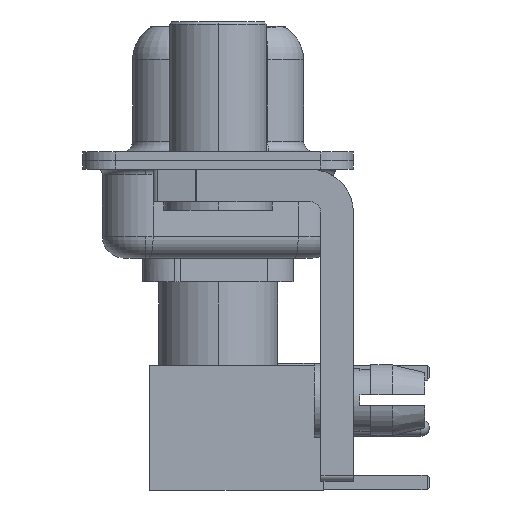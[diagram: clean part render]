
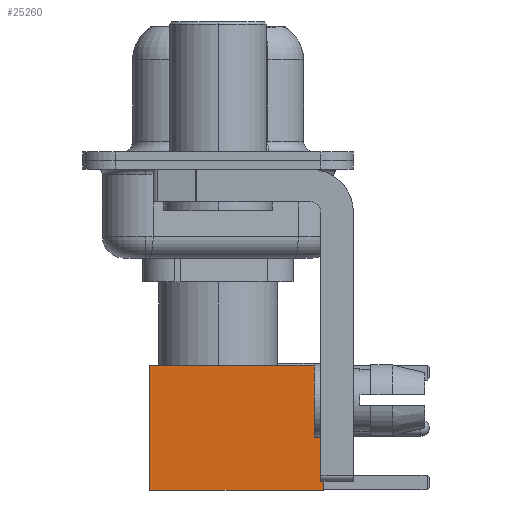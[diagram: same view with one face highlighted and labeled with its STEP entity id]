
A CAD part, left-side view. The second image highlights one B-rep face of the part: STEP entity #25260.
In plain terms, the highlighted face is planar.
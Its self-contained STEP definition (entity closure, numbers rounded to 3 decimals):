
#2645 = ORIENTED_EDGE ( 'NONE', *, *, #20282, .T. ) ;
#3722 = LINE ( 'NONE', #12527, #17031 ) ;
#4280 = CARTESIAN_POINT ( 'NONE',  ( 2.875, 2.875, 0. ) ) ;
#4749 = EDGE_CURVE ( 'NONE', #17745, #22793, #21740, .T. ) ;
#5296 = CARTESIAN_POINT ( 'NONE',  ( -2.875, 2.875, 8. ) ) ;
#5367 = CARTESIAN_POINT ( 'NONE',  ( 2.875, 2.875, 0. ) ) ;
#5919 = FACE_OUTER_BOUND ( 'NONE', #9492, .T. ) ;
#6090 = DIRECTION ( 'NONE',  ( 0., 0., -1. ) ) ;
#7211 = DIRECTION ( 'NONE',  ( -1., 0., 0. ) ) ;
#8745 = DIRECTION ( 'NONE',  ( 0., 0., 1. ) ) ;
#9492 = EDGE_LOOP ( 'NONE', ( #13717, #2645, #17162, #9732 ) ) ;
#9615 = EDGE_CURVE ( 'NONE', #10635, #19269, #24761, .T. ) ;
#9732 = ORIENTED_EDGE ( 'NONE', *, *, #21240, .F. ) ;
#9874 = CARTESIAN_POINT ( 'NONE',  ( 2.875, 2.875, 8. ) ) ;
#10264 = AXIS2_PLACEMENT_3D ( 'NONE', #5367, #14451, #8745 ) ;
#10635 = VERTEX_POINT ( 'NONE', #9874 ) ;
#12228 = VECTOR ( 'NONE', #6090, 1000. ) ;
#12253 = CARTESIAN_POINT ( 'NONE',  ( -2.875, 2.875, 0. ) ) ;
#12527 = CARTESIAN_POINT ( 'NONE',  ( 0., 2.875, 8. ) ) ;
#13603 = CARTESIAN_POINT ( 'NONE',  ( 0., 2.875, 0. ) ) ;
#13717 = ORIENTED_EDGE ( 'NONE', *, *, #9615, .T. ) ;
#14451 = DIRECTION ( 'NONE',  ( 0., 1., 0. ) ) ;
#15535 = CARTESIAN_POINT ( 'NONE',  ( -2.875, 2.875, 0. ) ) ;
#17031 = VECTOR ( 'NONE', #21645, 1000. ) ;
#17162 = ORIENTED_EDGE ( 'NONE', *, *, #4749, .F. ) ;
#17745 = VERTEX_POINT ( 'NONE', #5296 ) ;
#19269 = VERTEX_POINT ( 'NONE', #26663 ) ;
#20282 = EDGE_CURVE ( 'NONE', #19269, #22793, #27384, .T. ) ;
#21240 = EDGE_CURVE ( 'NONE', #10635, #17745, #3722, .T. ) ;
#21645 = DIRECTION ( 'NONE',  ( -1., 0., 0. ) ) ;
#21740 = LINE ( 'NONE', #15535, #22305 ) ;
#22305 = VECTOR ( 'NONE', #24544, 1000. ) ;
#22793 = VERTEX_POINT ( 'NONE', #12253 ) ;
#24544 = DIRECTION ( 'NONE',  ( 0., 0., -1. ) ) ;
#24761 = LINE ( 'NONE', #4280, #12228 ) ;
#25260 = ADVANCED_FACE ( 'NONE', ( #5919 ), #26826, .T. ) ;
#26663 = CARTESIAN_POINT ( 'NONE',  ( 2.875, 2.875, 0. ) ) ;
#26826 = PLANE ( 'NONE',  #10264 ) ;
#27384 = LINE ( 'NONE', #13603, #28480 ) ;
#28480 = VECTOR ( 'NONE', #7211, 1000. ) ;
